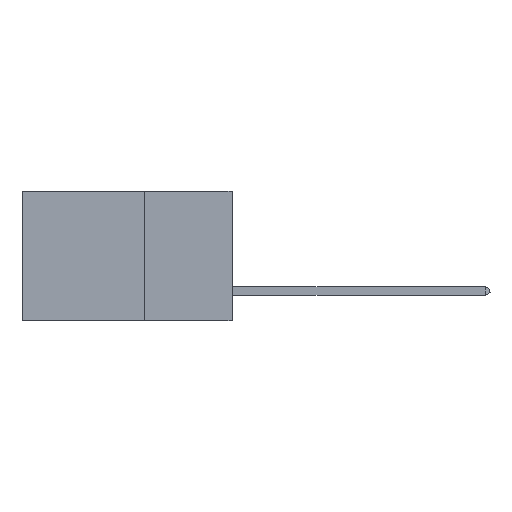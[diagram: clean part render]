
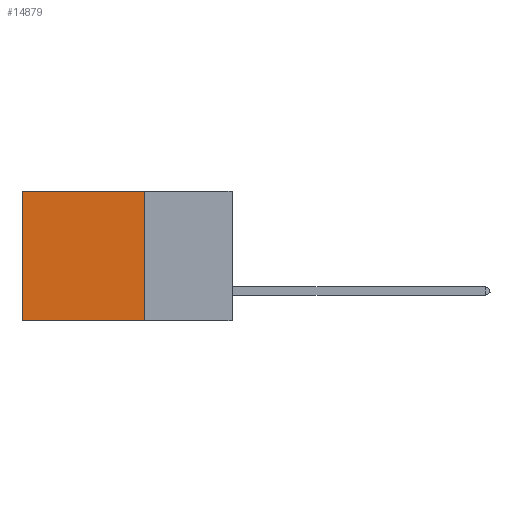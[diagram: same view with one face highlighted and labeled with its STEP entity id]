
A CAD part, left-side view. The second image highlights one B-rep face of the part: STEP entity #14879.
In plain terms, the highlighted planar face has unit normal (-1, 0, 0).
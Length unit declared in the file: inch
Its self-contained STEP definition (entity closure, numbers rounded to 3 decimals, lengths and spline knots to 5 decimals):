
#450 = EDGE_CURVE ( 'NONE', #20471, #5776, #1197, .T. ) ;
#1053 = CARTESIAN_POINT ( 'NONE',  ( 0.2875, 0.25, 0. ) ) ;
#1197 = LINE ( 'NONE', #2170, #6990 ) ;
#1920 = EDGE_CURVE ( 'NONE', #6536, #7082, #8338, .T. ) ;
#1949 = DIRECTION ( 'NONE',  ( 0., 0., -1. ) ) ;
#2170 = CARTESIAN_POINT ( 'NONE',  ( 0.2875, 0.25, 0. ) ) ;
#3439 = CARTESIAN_POINT ( 'NONE',  ( 0.2875, 0.25, 0. ) ) ;
#3471 = VECTOR ( 'NONE', #8977, 39.37008 ) ;
#3609 = ORIENTED_EDGE ( 'NONE', *, *, #1920, .T. ) ;
#4019 = CARTESIAN_POINT ( 'NONE',  ( 0.2875, 0.6, 0. ) ) ;
#5203 = VECTOR ( 'NONE', #15549, 39.37008 ) ;
#5776 = VERTEX_POINT ( 'NONE', #15851 ) ;
#6536 = VERTEX_POINT ( 'NONE', #19293 ) ;
#6830 = EDGE_LOOP ( 'NONE', ( #3609, #15950, #13738, #16335 ) ) ;
#6990 = VECTOR ( 'NONE', #1949, 39.37008 ) ;
#7082 = VERTEX_POINT ( 'NONE', #14439 ) ;
#7340 = AXIS2_PLACEMENT_3D ( 'NONE', #1053, #14620, #18074 ) ;
#7824 = PLANE ( 'NONE',  #7340 ) ;
#8338 = LINE ( 'NONE', #4019, #5203 ) ;
#8745 = EDGE_CURVE ( 'NONE', #5776, #7082, #19611, .T. ) ;
#8886 = CARTESIAN_POINT ( 'NONE',  ( 0.2875, 0.25, -0.37 ) ) ;
#8977 = DIRECTION ( 'NONE',  ( 0., 1., 0. ) ) ;
#10820 = LINE ( 'NONE', #18819, #3471 ) ;
#12029 = VECTOR ( 'NONE', #12268, 39.37008 ) ;
#12268 = DIRECTION ( 'NONE',  ( 0., 1., 0. ) ) ;
#13622 = FACE_OUTER_BOUND ( 'NONE', #6830, .T. ) ;
#13738 = ORIENTED_EDGE ( 'NONE', *, *, #450, .F. ) ;
#14439 = CARTESIAN_POINT ( 'NONE',  ( 0.2875, 0.6, -0.37 ) ) ;
#14620 = DIRECTION ( 'NONE',  ( 1., 0., 0. ) ) ;
#14879 = ADVANCED_FACE ( 'NONE', ( #13622 ), #7824, .F. ) ;
#15549 = DIRECTION ( 'NONE',  ( 0., 0., -1. ) ) ;
#15851 = CARTESIAN_POINT ( 'NONE',  ( 0.2875, 0.25, -0.37 ) ) ;
#15950 = ORIENTED_EDGE ( 'NONE', *, *, #8745, .F. ) ;
#16335 = ORIENTED_EDGE ( 'NONE', *, *, #20155, .T. ) ;
#18074 = DIRECTION ( 'NONE',  ( 0., 0., -1. ) ) ;
#18819 = CARTESIAN_POINT ( 'NONE',  ( 0.2875, 0.25, 0. ) ) ;
#19293 = CARTESIAN_POINT ( 'NONE',  ( 0.2875, 0.6, 0. ) ) ;
#19611 = LINE ( 'NONE', #8886, #12029 ) ;
#20155 = EDGE_CURVE ( 'NONE', #20471, #6536, #10820, .T. ) ;
#20471 = VERTEX_POINT ( 'NONE', #3439 ) ;
